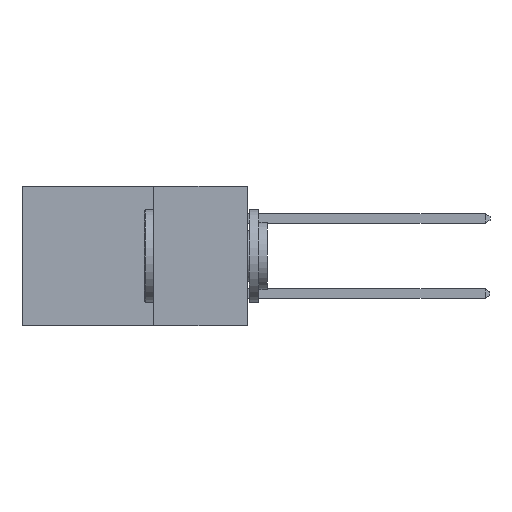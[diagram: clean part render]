
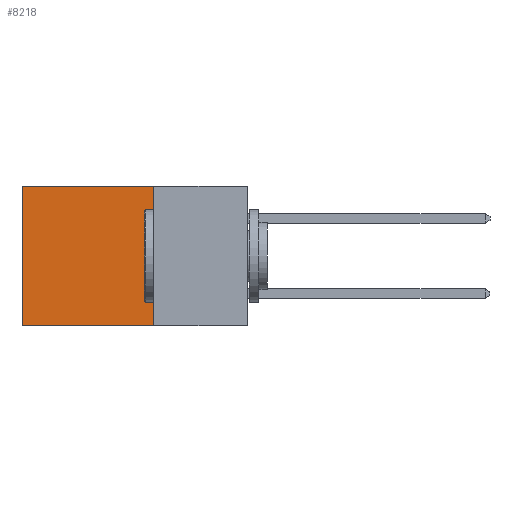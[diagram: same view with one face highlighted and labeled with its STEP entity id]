
A CAD part, left-side view. The second image highlights one B-rep face of the part: STEP entity #8218.
In plain terms, the highlighted planar face has unit normal (-1, 0, 0).
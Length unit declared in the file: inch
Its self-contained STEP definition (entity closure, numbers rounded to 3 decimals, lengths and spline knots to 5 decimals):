
#95 = DIRECTION ( 'NONE',  ( 0., 0., -1. ) ) ;
#199 = EDGE_CURVE ( 'NONE', #2978, #2282, #20144, .T. ) ;
#512 = DIRECTION ( 'NONE',  ( 0., 1., 0. ) ) ;
#1364 = EDGE_LOOP ( 'NONE', ( #8874, #19296, #17337, #14060 ) ) ;
#1537 = CARTESIAN_POINT ( 'NONE',  ( 0.298, 0.25, 0. ) ) ;
#1587 = CARTESIAN_POINT ( 'NONE',  ( 0.298, 0.6, 0. ) ) ;
#1843 = VECTOR ( 'NONE', #512, 39.37008 ) ;
#2144 = CARTESIAN_POINT ( 'NONE',  ( 0.298, 0.25, -0.37 ) ) ;
#2282 = VERTEX_POINT ( 'NONE', #3341 ) ;
#2852 = LINE ( 'NONE', #1537, #11417 ) ;
#2978 = VERTEX_POINT ( 'NONE', #7734 ) ;
#3266 = DIRECTION ( 'NONE',  ( 0., 0., -1. ) ) ;
#3341 = CARTESIAN_POINT ( 'NONE',  ( 0.298, 0.6, -0.37 ) ) ;
#4269 = CARTESIAN_POINT ( 'NONE',  ( 0.298, 0.25, 0. ) ) ;
#5160 = CARTESIAN_POINT ( 'NONE',  ( 0.298, 0.25, 0. ) ) ;
#5347 = VECTOR ( 'NONE', #9456, 39.37008 ) ;
#7697 = CARTESIAN_POINT ( 'NONE',  ( 0.298, 0.6, 0. ) ) ;
#7734 = CARTESIAN_POINT ( 'NONE',  ( 0.298, 0.25, -0.37 ) ) ;
#8218 = ADVANCED_FACE ( 'NONE', ( #18701 ), #21264, .F. ) ;
#8874 = ORIENTED_EDGE ( 'NONE', *, *, #16633, .T. ) ;
#9456 = DIRECTION ( 'NONE',  ( 0., 0., -1. ) ) ;
#10350 = DIRECTION ( 'NONE',  ( 0., 1., 0. ) ) ;
#11417 = VECTOR ( 'NONE', #3266, 39.37008 ) ;
#12064 = EDGE_CURVE ( 'NONE', #21660, #2978, #2852, .T. ) ;
#12392 = AXIS2_PLACEMENT_3D ( 'NONE', #4269, #16273, #95 ) ;
#12698 = VERTEX_POINT ( 'NONE', #1587 ) ;
#14060 = ORIENTED_EDGE ( 'NONE', *, *, #18266, .T. ) ;
#14971 = VECTOR ( 'NONE', #10350, 39.37008 ) ;
#16081 = LINE ( 'NONE', #5160, #14971 ) ;
#16273 = DIRECTION ( 'NONE',  ( 1., 0., 0. ) ) ;
#16633 = EDGE_CURVE ( 'NONE', #12698, #2282, #19105, .T. ) ;
#17337 = ORIENTED_EDGE ( 'NONE', *, *, #12064, .F. ) ;
#18266 = EDGE_CURVE ( 'NONE', #21660, #12698, #16081, .T. ) ;
#18501 = CARTESIAN_POINT ( 'NONE',  ( 0.298, 0.25, 0. ) ) ;
#18701 = FACE_OUTER_BOUND ( 'NONE', #1364, .T. ) ;
#19105 = LINE ( 'NONE', #7697, #5347 ) ;
#19296 = ORIENTED_EDGE ( 'NONE', *, *, #199, .F. ) ;
#20144 = LINE ( 'NONE', #2144, #1843 ) ;
#21264 = PLANE ( 'NONE',  #12392 ) ;
#21660 = VERTEX_POINT ( 'NONE', #18501 ) ;
